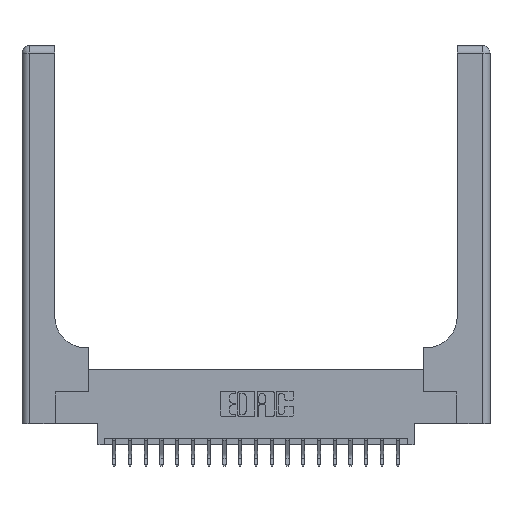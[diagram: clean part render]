
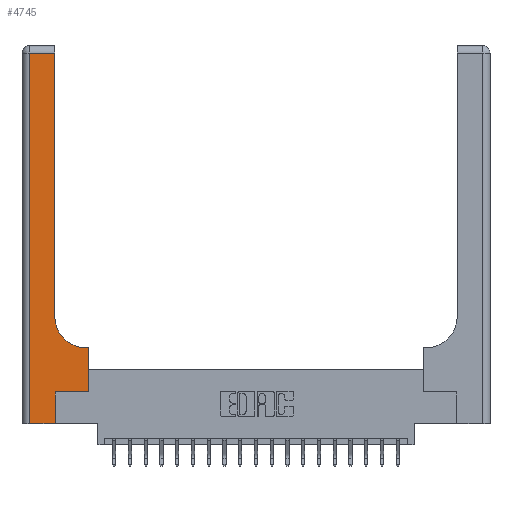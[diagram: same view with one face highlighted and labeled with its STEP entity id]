
A CAD part, top view. The second image highlights one B-rep face of the part: STEP entity #4745.
In plain terms, the highlighted planar face has unit normal (0, 0, 1).
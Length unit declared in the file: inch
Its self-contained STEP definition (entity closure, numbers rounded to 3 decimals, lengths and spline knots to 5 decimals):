
#5 = FACE_OUTER_BOUND ( 'NONE', #4322, .T. ) ;
#379 = VERTEX_POINT ( 'NONE', #18624 ) ;
#606 = EDGE_CURVE ( 'NONE', #3492, #4760, #8422, .T. ) ;
#817 = EDGE_CURVE ( 'NONE', #4760, #379, #15812, .T. ) ;
#887 = CARTESIAN_POINT ( 'NONE',  ( 0.51, 0.85, 0.37 ) ) ;
#1012 = LINE ( 'NONE', #7760, #2785 ) ;
#1058 = CARTESIAN_POINT ( 'NONE',  ( 0.528, 0.6, 0.37 ) ) ;
#1129 = VECTOR ( 'NONE', #14673, 39.37008 ) ;
#1190 = LINE ( 'NONE', #12941, #12596 ) ;
#1651 = VECTOR ( 'NONE', #5916, 39.37008 ) ;
#2499 = VECTOR ( 'NONE', #18242, 39.37008 ) ;
#2785 = VECTOR ( 'NONE', #6132, 39.37008 ) ;
#2824 = ORIENTED_EDGE ( 'NONE', *, *, #11669, .T. ) ;
#3168 = ORIENTED_EDGE ( 'NONE', *, *, #817, .T. ) ;
#3442 = CARTESIAN_POINT ( 'NONE',  ( 0.26, 0.6, 0.37 ) ) ;
#3492 = VERTEX_POINT ( 'NONE', #11142 ) ;
#3683 = VERTEX_POINT ( 'NONE', #16883 ) ;
#3938 = DIRECTION ( 'NONE',  ( -1., 0., 0. ) ) ;
#4322 = EDGE_LOOP ( 'NONE', ( #6041, #4456, #9322, #3168, #21275, #20001, #6502, #4612, #2824 ) ) ;
#4456 = ORIENTED_EDGE ( 'NONE', *, *, #12170, .T. ) ;
#4612 = ORIENTED_EDGE ( 'NONE', *, *, #19965, .T. ) ;
#4745 = ADVANCED_FACE ( 'NONE', ( #5 ), #6647, .F. ) ;
#4760 = VERTEX_POINT ( 'NONE', #11756 ) ;
#5091 = VERTEX_POINT ( 'NONE', #13151 ) ;
#5592 = CARTESIAN_POINT ( 'NONE',  ( 0., 0., 0.37 ) ) ;
#5916 = DIRECTION ( 'NONE',  ( 1., 0., 0. ) ) ;
#6041 = ORIENTED_EDGE ( 'NONE', *, *, #14981, .T. ) ;
#6132 = DIRECTION ( 'NONE',  ( 1., 0., 0. ) ) ;
#6502 = ORIENTED_EDGE ( 'NONE', *, *, #15089, .T. ) ;
#6647 = PLANE ( 'NONE',  #16292 ) ;
#6652 = VERTEX_POINT ( 'NONE', #1058 ) ;
#6808 = DIRECTION ( 'NONE',  ( -1., 0., 0. ) ) ;
#7340 = CIRCLE ( 'NONE', #20526, 0.25 ) ;
#7457 = DIRECTION ( 'NONE',  ( 0., 1., 0. ) ) ;
#7525 = DIRECTION ( 'NONE',  ( 0., 0., -1. ) ) ;
#7760 = CARTESIAN_POINT ( 'NONE',  ( 0.265, 0.25, 0.37 ) ) ;
#7929 = DIRECTION ( 'NONE',  ( 0., 1., 0. ) ) ;
#8245 = VECTOR ( 'NONE', #14943, 39.37008 ) ;
#8422 = LINE ( 'NONE', #12001, #8245 ) ;
#9322 = ORIENTED_EDGE ( 'NONE', *, *, #606, .T. ) ;
#9358 = CARTESIAN_POINT ( 'NONE',  ( 0.528, 0.25, 0.37 ) ) ;
#9653 = CARTESIAN_POINT ( 'NONE',  ( 0., 2.94, 0.37 ) ) ;
#10036 = EDGE_CURVE ( 'NONE', #3683, #21279, #1012, .T. ) ;
#10293 = CARTESIAN_POINT ( 'NONE',  ( 0.265, 0., 0.37 ) ) ;
#11142 = CARTESIAN_POINT ( 'NONE',  ( 0.06, 2.94, 0.37 ) ) ;
#11395 = VECTOR ( 'NONE', #6808, 39.37008 ) ;
#11401 = LINE ( 'NONE', #9653, #2499 ) ;
#11669 = EDGE_CURVE ( 'NONE', #15421, #12497, #7340, .T. ) ;
#11756 = CARTESIAN_POINT ( 'NONE',  ( 0.06, 0., 0.37 ) ) ;
#12001 = CARTESIAN_POINT ( 'NONE',  ( 0.06, 3., 0.37 ) ) ;
#12170 = EDGE_CURVE ( 'NONE', #5091, #3492, #11401, .T. ) ;
#12497 = VERTEX_POINT ( 'NONE', #19618 ) ;
#12596 = VECTOR ( 'NONE', #7929, 39.37008 ) ;
#12941 = CARTESIAN_POINT ( 'NONE',  ( 0.26, 3., 0.37 ) ) ;
#13055 = DIRECTION ( 'NONE',  ( 1., 0., 0. ) ) ;
#13151 = CARTESIAN_POINT ( 'NONE',  ( 0.26, 2.94, 0.37 ) ) ;
#13294 = CARTESIAN_POINT ( 'NONE',  ( 0., 3., 0.37 ) ) ;
#14220 = CARTESIAN_POINT ( 'NONE',  ( 0.51, 0.6, 0.37 ) ) ;
#14556 = EDGE_CURVE ( 'NONE', #379, #3683, #17246, .T. ) ;
#14673 = DIRECTION ( 'NONE',  ( 0., 1., 0. ) ) ;
#14943 = DIRECTION ( 'NONE',  ( 0., -1., 0. ) ) ;
#14981 = EDGE_CURVE ( 'NONE', #12497, #5091, #1190, .T. ) ;
#15008 = VECTOR ( 'NONE', #7457, 39.37008 ) ;
#15082 = LINE ( 'NONE', #3442, #11395 ) ;
#15089 = EDGE_CURVE ( 'NONE', #21279, #6652, #18030, .T. ) ;
#15421 = VERTEX_POINT ( 'NONE', #14220 ) ;
#15812 = LINE ( 'NONE', #5592, #1651 ) ;
#16292 = AXIS2_PLACEMENT_3D ( 'NONE', #13294, #19907, #3938 ) ;
#16694 = CARTESIAN_POINT ( 'NONE',  ( 0.528, 0.25, 0.37 ) ) ;
#16883 = CARTESIAN_POINT ( 'NONE',  ( 0.265, 0.25, 0.37 ) ) ;
#17246 = LINE ( 'NONE', #10293, #15008 ) ;
#18030 = LINE ( 'NONE', #9358, #1129 ) ;
#18242 = DIRECTION ( 'NONE',  ( -1., 0., 0. ) ) ;
#18624 = CARTESIAN_POINT ( 'NONE',  ( 0.265, 0., 0.37 ) ) ;
#19618 = CARTESIAN_POINT ( 'NONE',  ( 0.26, 0.85, 0.37 ) ) ;
#19907 = DIRECTION ( 'NONE',  ( 0., 0., -1. ) ) ;
#19965 = EDGE_CURVE ( 'NONE', #6652, #15421, #15082, .T. ) ;
#20001 = ORIENTED_EDGE ( 'NONE', *, *, #10036, .T. ) ;
#20526 = AXIS2_PLACEMENT_3D ( 'NONE', #887, #7525, #13055 ) ;
#21275 = ORIENTED_EDGE ( 'NONE', *, *, #14556, .T. ) ;
#21279 = VERTEX_POINT ( 'NONE', #16694 ) ;
